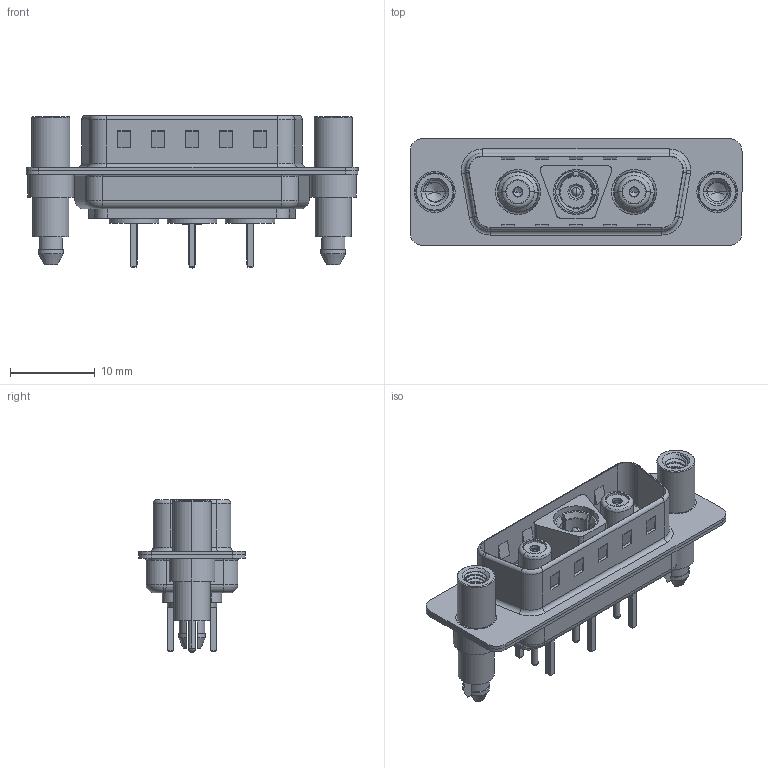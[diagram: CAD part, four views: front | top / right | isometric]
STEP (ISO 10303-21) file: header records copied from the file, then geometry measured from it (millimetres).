
FILE_DESCRIPTION (( 'STEP AP203' ), '1' );
FILE_NAME ('627-3WK3224-7NE.STEP', '2019-05-24T22:31:47', ( '' ), ( '' ), 'SwSTEP 2.0', 'SolidWorks 2016', '' );
FILE_SCHEMA (( 'CONFIG_CONTROL_DESIGN' ));
Length unit declared in the file: millimetre
Products named in the file (16): Locking Collar; Co-Ax Plug Assy_S; 627Combo Housing_3WK3; 627-3WK3224-7NE; Co-Ax Jack_Straight PC Tail; 627Combo Shell Rear_15 Contacts; Insulator Socket; 627Combo Shell Front_15 Contacts; Insulator Socket 2; 627Combo Threaded Standoff and Boardlock_E; Socket_Str; Co-Ax Plug_Straight PC Tail; Co-Ax Jack Assy_S; Insulator Pin_Straight PC Tail; 627Combo Threaded Standoff and Boardlock_6; Pin_Str
Assembly tree (17 placements, depth 3):
  627-3WK3224-7NE
    627Combo Housing_3WK3
    627Combo Shell Rear_15 Contacts
    627Combo Shell Front_15 Contacts
    627Combo Threaded Standoff and Boardlock_E
    Co-Ax Plug Assy_S
      Co-Ax Plug_Straight PC Tail
      Insulator Pin_Straight PC Tail
      Pin_Str
      Locking Collar
    Co-Ax Jack Assy_S  x2
      Co-Ax Jack_Straight PC Tail
      Insulator Socket
      Insulator Socket 2
      Locking Collar
      Socket_Str
    627Combo Threaded Standoff and Boardlock_6
Bounding box: 39.15 x 12.6 x 18 mm (x, y, z)
Volume: 2356.2 mm3; surface area: 6544.5 mm2
Topology: 19 solids, 19 shells, 754 faces, 1821 edges, 1147 vertices
Faces by surface type: plane 313, cylinder 309, torus 62, cone 50, bspline 12, sphere 8
Entity records: 22974 total; most frequent: CARTESIAN_POINT 5989, DIRECTION 3319, ORIENTED_EDGE 3094, EDGE_CURVE 1547, AXIS2_PLACEMENT_3D 1259, VERTEX_POINT 985, VECTOR 801, LINE 801
